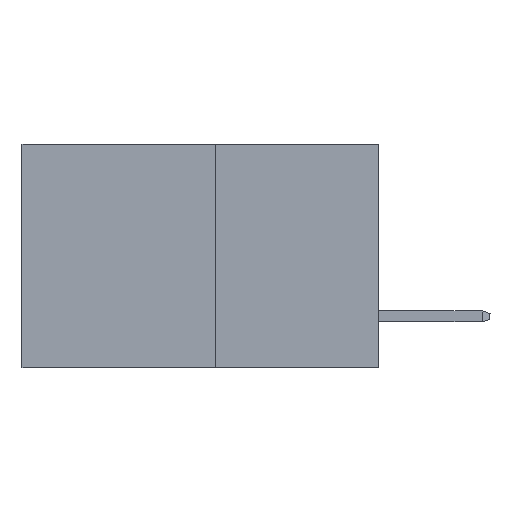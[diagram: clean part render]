
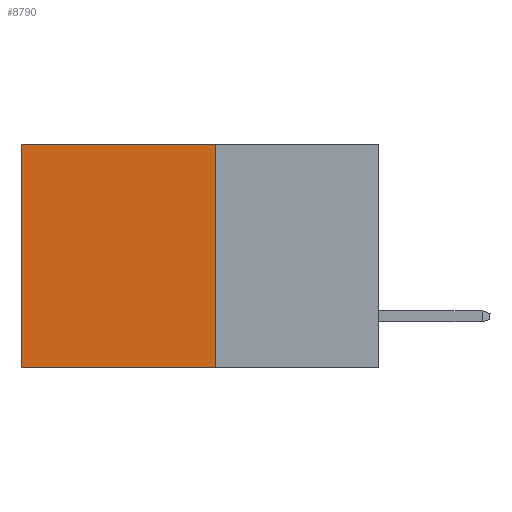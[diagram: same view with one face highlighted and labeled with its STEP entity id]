
A CAD part, left-side view. The second image highlights one B-rep face of the part: STEP entity #8790.
In plain terms, the highlighted planar face has unit normal (-1, 0, 0).
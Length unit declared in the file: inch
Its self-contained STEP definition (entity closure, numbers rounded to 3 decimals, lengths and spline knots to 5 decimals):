
#284 = EDGE_CURVE ( 'NONE', #7007, #4795, #3383, .T. ) ;
#761 = EDGE_CURVE ( 'NONE', #4795, #5760, #859, .T. ) ;
#859 = LINE ( 'NONE', #4386, #5261 ) ;
#1278 = EDGE_CURVE ( 'NONE', #6226, #5760, #1290, .T. ) ;
#1290 = LINE ( 'NONE', #5185, #5634 ) ;
#2316 = CARTESIAN_POINT ( 'NONE',  ( 0.277, 0.27, -0.37 ) ) ;
#2695 = PLANE ( 'NONE',  #5897 ) ;
#2781 = DIRECTION ( 'NONE',  ( 0., 1., 0. ) ) ;
#3383 = LINE ( 'NONE', #8517, #7696 ) ;
#3929 = CARTESIAN_POINT ( 'NONE',  ( 0.277, 0.59, 0. ) ) ;
#4199 = DIRECTION ( 'NONE',  ( 0., 0., -1. ) ) ;
#4257 = FACE_OUTER_BOUND ( 'NONE', #4936, .T. ) ;
#4341 = CARTESIAN_POINT ( 'NONE',  ( 0.277, 0.59, -0.37 ) ) ;
#4377 = DIRECTION ( 'NONE',  ( 0., 0., -1. ) ) ;
#4386 = CARTESIAN_POINT ( 'NONE',  ( 0.277, 0.59, -0.37 ) ) ;
#4430 = CARTESIAN_POINT ( 'NONE',  ( 0.277, 0.27, -0.37 ) ) ;
#4795 = VERTEX_POINT ( 'NONE', #3929 ) ;
#4936 = EDGE_LOOP ( 'NONE', ( #5127, #5467, #5555, #5716 ) ) ;
#5127 = ORIENTED_EDGE ( 'NONE', *, *, #761, .T. ) ;
#5185 = CARTESIAN_POINT ( 'NONE',  ( 0.277, 0.27, -0.37 ) ) ;
#5245 = EDGE_CURVE ( 'NONE', #7007, #6226, #5329, .T. ) ;
#5261 = VECTOR ( 'NONE', #4199, 39.37008 ) ;
#5329 = LINE ( 'NONE', #4430, #7197 ) ;
#5467 = ORIENTED_EDGE ( 'NONE', *, *, #1278, .F. ) ;
#5555 = ORIENTED_EDGE ( 'NONE', *, *, #5245, .F. ) ;
#5634 = VECTOR ( 'NONE', #7093, 39.37008 ) ;
#5716 = ORIENTED_EDGE ( 'NONE', *, *, #284, .T. ) ;
#5760 = VERTEX_POINT ( 'NONE', #4341 ) ;
#5897 = AXIS2_PLACEMENT_3D ( 'NONE', #7592, #9162, #4377 ) ;
#6226 = VERTEX_POINT ( 'NONE', #2316 ) ;
#6865 = DIRECTION ( 'NONE',  ( 0., 0., -1. ) ) ;
#7007 = VERTEX_POINT ( 'NONE', #10199 ) ;
#7093 = DIRECTION ( 'NONE',  ( 0., 1., 0. ) ) ;
#7197 = VECTOR ( 'NONE', #6865, 39.37008 ) ;
#7592 = CARTESIAN_POINT ( 'NONE',  ( 0.277, 0.27, -0.37 ) ) ;
#7696 = VECTOR ( 'NONE', #2781, 39.37008 ) ;
#8517 = CARTESIAN_POINT ( 'NONE',  ( 0.277, 0.27, 0. ) ) ;
#8790 = ADVANCED_FACE ( 'NONE', ( #4257 ), #2695, .F. ) ;
#9162 = DIRECTION ( 'NONE',  ( 1., 0., 0. ) ) ;
#10199 = CARTESIAN_POINT ( 'NONE',  ( 0.277, 0.27, 0. ) ) ;
